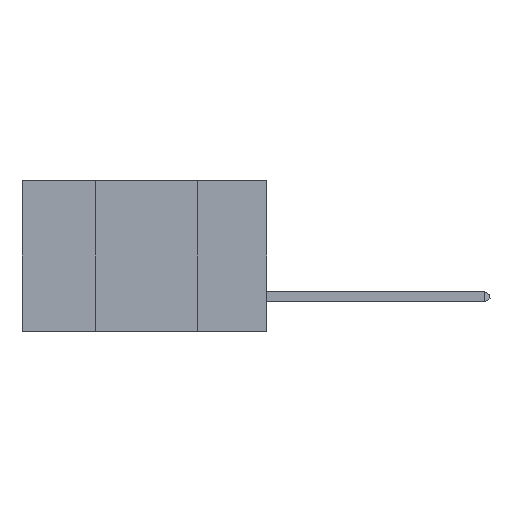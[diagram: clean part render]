
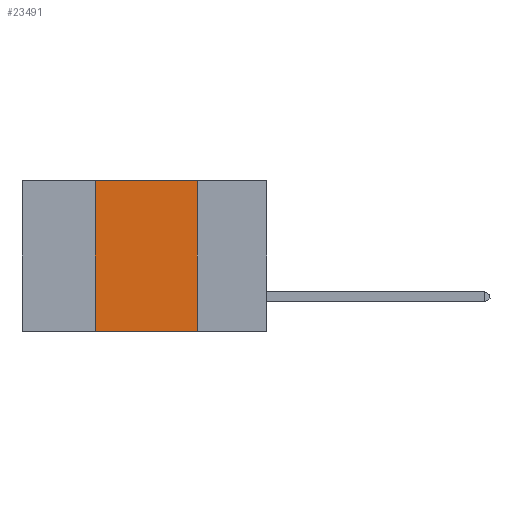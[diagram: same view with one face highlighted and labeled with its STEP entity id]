
A CAD part, left-side view. The second image highlights one B-rep face of the part: STEP entity #23491.
In plain terms, the highlighted planar face has unit normal (-1, 0, 0).
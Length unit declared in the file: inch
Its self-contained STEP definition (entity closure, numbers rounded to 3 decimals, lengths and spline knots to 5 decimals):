
#3490 = DIRECTION ( 'NONE',  ( 0., 0., -1. ) ) ;
#3893 = ORIENTED_EDGE ( 'NONE', *, *, #30426, .F. ) ;
#4404 = LINE ( 'NONE', #18044, #19850 ) ;
#4740 = EDGE_CURVE ( 'NONE', #15363, #7402, #13674, .T. ) ;
#5499 = VECTOR ( 'NONE', #31263, 39.37008 ) ;
#7402 = VERTEX_POINT ( 'NONE', #20714 ) ;
#8468 = CARTESIAN_POINT ( 'NONE',  ( 0., 0.6, 0. ) ) ;
#9640 = VECTOR ( 'NONE', #21921, 39.37008 ) ;
#11996 = CARTESIAN_POINT ( 'NONE',  ( 0., 0.42, -0.37 ) ) ;
#12665 = CARTESIAN_POINT ( 'NONE',  ( 0., 0.6, 0. ) ) ;
#13015 = CARTESIAN_POINT ( 'NONE',  ( 0., 0.17, 0. ) ) ;
#13674 = LINE ( 'NONE', #13015, #5499 ) ;
#14147 = LINE ( 'NONE', #8468, #36521 ) ;
#15363 = VERTEX_POINT ( 'NONE', #31921 ) ;
#16503 = EDGE_CURVE ( 'NONE', #34603, #7402, #26821, .T. ) ;
#18044 = CARTESIAN_POINT ( 'NONE',  ( 0., 0.42, 0. ) ) ;
#18893 = PLANE ( 'NONE',  #37133 ) ;
#19850 = VECTOR ( 'NONE', #39266, 39.37008 ) ;
#20714 = CARTESIAN_POINT ( 'NONE',  ( 0., 0.17, -0.37 ) ) ;
#21921 = DIRECTION ( 'NONE',  ( 0., -1., 0. ) ) ;
#21940 = DIRECTION ( 'NONE',  ( 1., 0., 0. ) ) ;
#23137 = ORIENTED_EDGE ( 'NONE', *, *, #16503, .T. ) ;
#23491 = ADVANCED_FACE ( 'NONE', ( #37907 ), #18893, .F. ) ;
#23561 = CARTESIAN_POINT ( 'NONE',  ( 0., 0.42, 0. ) ) ;
#23952 = EDGE_CURVE ( 'NONE', #34603, #28776, #4404, .T. ) ;
#25886 = EDGE_LOOP ( 'NONE', ( #31584, #3893, #28319, #23137 ) ) ;
#26754 = DIRECTION ( 'NONE',  ( 0., -1., 0. ) ) ;
#26821 = LINE ( 'NONE', #37027, #9640 ) ;
#28319 = ORIENTED_EDGE ( 'NONE', *, *, #23952, .F. ) ;
#28776 = VERTEX_POINT ( 'NONE', #23561 ) ;
#30426 = EDGE_CURVE ( 'NONE', #28776, #15363, #14147, .T. ) ;
#31263 = DIRECTION ( 'NONE',  ( 0., 0., -1. ) ) ;
#31584 = ORIENTED_EDGE ( 'NONE', *, *, #4740, .F. ) ;
#31921 = CARTESIAN_POINT ( 'NONE',  ( 0., 0.17, 0. ) ) ;
#34603 = VERTEX_POINT ( 'NONE', #11996 ) ;
#36521 = VECTOR ( 'NONE', #26754, 39.37008 ) ;
#37027 = CARTESIAN_POINT ( 'NONE',  ( 0., 0.6, -0.37 ) ) ;
#37133 = AXIS2_PLACEMENT_3D ( 'NONE', #12665, #21940, #3490 ) ;
#37907 = FACE_OUTER_BOUND ( 'NONE', #25886, .T. ) ;
#39266 = DIRECTION ( 'NONE',  ( 0., 0., 1. ) ) ;
